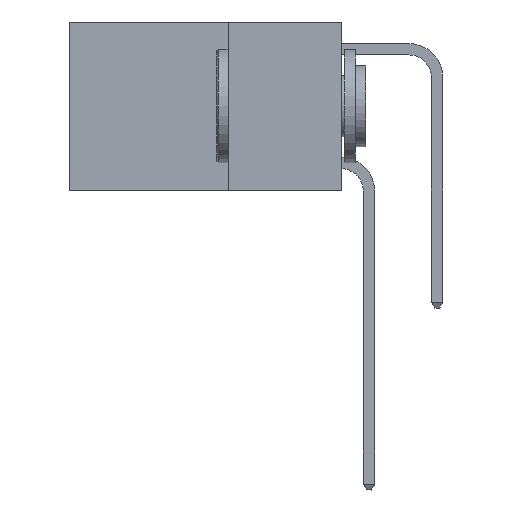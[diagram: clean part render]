
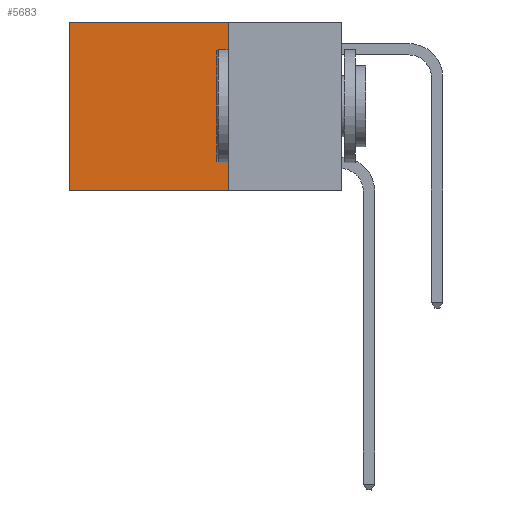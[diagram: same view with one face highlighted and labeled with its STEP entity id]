
A CAD part, left-side view. The second image highlights one B-rep face of the part: STEP entity #5683.
In plain terms, the highlighted planar face has unit normal (-1, 0, 0).
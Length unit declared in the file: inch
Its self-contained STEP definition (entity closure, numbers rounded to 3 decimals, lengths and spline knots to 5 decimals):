
#195 = EDGE_LOOP ( 'NONE', ( #7484, #10192, #12737, #13038 ) ) ;
#381 = LINE ( 'NONE', #10832, #11412 ) ;
#585 = VECTOR ( 'NONE', #9083, 39.37008 ) ;
#918 = DIRECTION ( 'NONE',  ( 1., 0., 0. ) ) ;
#1263 = DIRECTION ( 'NONE',  ( 0., 0., -1. ) ) ;
#1660 = VERTEX_POINT ( 'NONE', #6869 ) ;
#2607 = DIRECTION ( 'NONE',  ( 0., 1., 0. ) ) ;
#2641 = CARTESIAN_POINT ( 'NONE',  ( 0.2625, 0.6, 0. ) ) ;
#4535 = FACE_OUTER_BOUND ( 'NONE', #195, .T. ) ;
#4917 = EDGE_CURVE ( 'NONE', #5475, #7689, #10774, .T. ) ;
#5072 = CARTESIAN_POINT ( 'NONE',  ( 0.2625, 0.25, 0. ) ) ;
#5394 = CARTESIAN_POINT ( 'NONE',  ( 0.2625, 0.25, -0.37 ) ) ;
#5475 = VERTEX_POINT ( 'NONE', #2641 ) ;
#5602 = EDGE_CURVE ( 'NONE', #13128, #7689, #10919, .T. ) ;
#5683 = ADVANCED_FACE ( 'NONE', ( #4535 ), #6139, .F. ) ;
#6139 = PLANE ( 'NONE',  #13516 ) ;
#6168 = LINE ( 'NONE', #5072, #585 ) ;
#6869 = CARTESIAN_POINT ( 'NONE',  ( 0.2625, 0.25, 0. ) ) ;
#6997 = DIRECTION ( 'NONE',  ( 0., 1., 0. ) ) ;
#7484 = ORIENTED_EDGE ( 'NONE', *, *, #4917, .T. ) ;
#7689 = VERTEX_POINT ( 'NONE', #10484 ) ;
#8140 = DIRECTION ( 'NONE',  ( 0., 0., -1. ) ) ;
#8163 = VECTOR ( 'NONE', #6997, 39.37008 ) ;
#9003 = CARTESIAN_POINT ( 'NONE',  ( 0.2625, 0.25, -0.37 ) ) ;
#9083 = DIRECTION ( 'NONE',  ( 0., 0., -1. ) ) ;
#10159 = CARTESIAN_POINT ( 'NONE',  ( 0.2625, 0.25, 0. ) ) ;
#10192 = ORIENTED_EDGE ( 'NONE', *, *, #5602, .F. ) ;
#10484 = CARTESIAN_POINT ( 'NONE',  ( 0.2625, 0.6, -0.37 ) ) ;
#10774 = LINE ( 'NONE', #12646, #11100 ) ;
#10832 = CARTESIAN_POINT ( 'NONE',  ( 0.2625, 0.25, 0. ) ) ;
#10870 = EDGE_CURVE ( 'NONE', #1660, #13128, #6168, .T. ) ;
#10919 = LINE ( 'NONE', #9003, #8163 ) ;
#11100 = VECTOR ( 'NONE', #1263, 39.37008 ) ;
#11412 = VECTOR ( 'NONE', #2607, 39.37008 ) ;
#12646 = CARTESIAN_POINT ( 'NONE',  ( 0.2625, 0.6, 0. ) ) ;
#12712 = EDGE_CURVE ( 'NONE', #1660, #5475, #381, .T. ) ;
#12737 = ORIENTED_EDGE ( 'NONE', *, *, #10870, .F. ) ;
#13038 = ORIENTED_EDGE ( 'NONE', *, *, #12712, .T. ) ;
#13128 = VERTEX_POINT ( 'NONE', #5394 ) ;
#13516 = AXIS2_PLACEMENT_3D ( 'NONE', #10159, #918, #8140 ) ;
